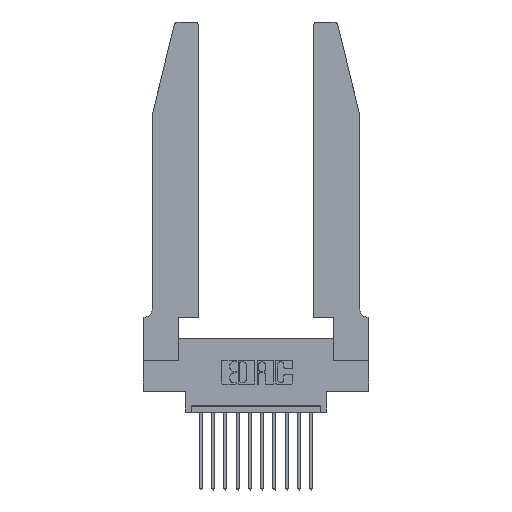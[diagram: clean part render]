
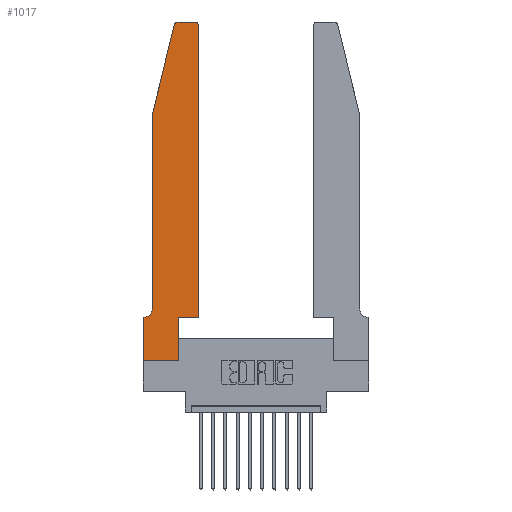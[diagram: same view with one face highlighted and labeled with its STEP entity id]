
A CAD part, top view. The second image highlights one B-rep face of the part: STEP entity #1017.
In plain terms, the highlighted planar face has unit normal (0, 0, 1).
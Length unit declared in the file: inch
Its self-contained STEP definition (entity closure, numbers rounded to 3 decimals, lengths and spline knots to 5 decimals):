
#287 = EDGE_CURVE ( 'NONE', #5123, #6462, #5227, .T. ) ;
#562 = EDGE_CURVE ( 'NONE', #6462, #10882, #5429, .T. ) ;
#591 = LINE ( 'NONE', #732, #14550 ) ;
#655 = LINE ( 'NONE', #1551, #4544 ) ;
#732 = CARTESIAN_POINT ( 'NONE',  ( 0.0755, 2., 0.37 ) ) ;
#905 = ORIENTED_EDGE ( 'NONE', *, *, #12483, .T. ) ;
#939 = ORIENTED_EDGE ( 'NONE', *, *, #8264, .T. ) ;
#1017 = ADVANCED_FACE ( 'NONE', ( #9072 ), #1967, .T. ) ;
#1148 = DIRECTION ( 'NONE',  ( -1., 0., 0. ) ) ;
#1418 = EDGE_CURVE ( 'NONE', #13668, #5212, #11691, .T. ) ;
#1441 = ORIENTED_EDGE ( 'NONE', *, *, #1418, .T. ) ;
#1551 = CARTESIAN_POINT ( 'NONE',  ( 0., 0., 0.37 ) ) ;
#1609 = ORIENTED_EDGE ( 'NONE', *, *, #4348, .T. ) ;
#1967 = PLANE ( 'NONE',  #3558 ) ;
#2048 = CARTESIAN_POINT ( 'NONE',  ( 0.0755, 2., 0.37 ) ) ;
#2219 = EDGE_CURVE ( 'NONE', #9924, #5123, #9487, .T. ) ;
#2852 = DIRECTION ( 'NONE',  ( 0., -1., 0. ) ) ;
#2878 = EDGE_LOOP ( 'NONE', ( #8691, #9067, #11503, #939, #1609, #10460, #5895, #1441, #905, #11869, #11706, #11592 ) ) ;
#2942 = CARTESIAN_POINT ( 'NONE',  ( 0.284, 2.75, 0.37 ) ) ;
#3267 = DIRECTION ( 'NONE',  ( 1., 0., 0. ) ) ;
#3558 = AXIS2_PLACEMENT_3D ( 'NONE', #5874, #7363, #3267 ) ;
#4331 = DIRECTION ( 'NONE',  ( 0., 0., 1. ) ) ;
#4348 = EDGE_CURVE ( 'NONE', #7393, #15270, #9015, .T. ) ;
#4485 = CARTESIAN_POINT ( 'NONE',  ( 0.4505, 0.35, 0.37 ) ) ;
#4508 = DIRECTION ( 'NONE',  ( 1., 0., 0. ) ) ;
#4544 = VECTOR ( 'NONE', #2852, 39.37008 ) ;
#4718 = CARTESIAN_POINT ( 'NONE',  ( 0.0755, 0.35, 0.37 ) ) ;
#4980 = CARTESIAN_POINT ( 'NONE',  ( 0.0055, 0.42, 0.37 ) ) ;
#5123 = VERTEX_POINT ( 'NONE', #12756 ) ;
#5212 = VERTEX_POINT ( 'NONE', #10703 ) ;
#5227 = LINE ( 'NONE', #4485, #16720 ) ;
#5264 = CARTESIAN_POINT ( 'NONE',  ( 0.4205, 2.72, 0.37 ) ) ;
#5366 = CARTESIAN_POINT ( 'NONE',  ( 0., 0.35, 0.37 ) ) ;
#5429 = CIRCLE ( 'NONE', #11139, 0.03 ) ;
#5450 = CARTESIAN_POINT ( 'NONE',  ( 0.2865, 0.35, 0.37 ) ) ;
#5461 = DIRECTION ( 'NONE',  ( 0., 1., 0. ) ) ;
#5874 = CARTESIAN_POINT ( 'NONE',  ( 0., 0.35, 0.37 ) ) ;
#5892 = VERTEX_POINT ( 'NONE', #5366 ) ;
#5895 = ORIENTED_EDGE ( 'NONE', *, *, #12317, .T. ) ;
#6407 = CARTESIAN_POINT ( 'NONE',  ( 0.0055, 0.35, 0.37 ) ) ;
#6462 = VERTEX_POINT ( 'NONE', #16667 ) ;
#6620 = DIRECTION ( 'NONE',  ( -0.239, -0.971, 0. ) ) ;
#6902 = CARTESIAN_POINT ( 'NONE',  ( 0., 0., 0.37 ) ) ;
#7152 = EDGE_CURVE ( 'NONE', #15270, #5892, #15324, .T. ) ;
#7336 = CARTESIAN_POINT ( 'NONE',  ( 0.25487, 2.72718, 0.37 ) ) ;
#7363 = DIRECTION ( 'NONE',  ( 0., 0., 1. ) ) ;
#7393 = VERTEX_POINT ( 'NONE', #14456 ) ;
#7617 = DIRECTION ( 'NONE',  ( 0., 0., -1. ) ) ;
#8003 = DIRECTION ( 'NONE',  ( 1., 0., 0. ) ) ;
#8075 = EDGE_CURVE ( 'NONE', #8812, #16035, #8946, .T. ) ;
#8092 = CARTESIAN_POINT ( 'NONE',  ( 0., 0., 0.37 ) ) ;
#8264 = EDGE_CURVE ( 'NONE', #9399, #7393, #591, .T. ) ;
#8691 = ORIENTED_EDGE ( 'NONE', *, *, #10604, .T. ) ;
#8812 = VERTEX_POINT ( 'NONE', #2942 ) ;
#8946 = CIRCLE ( 'NONE', #13053, 0.03 ) ;
#9015 = CIRCLE ( 'NONE', #10762, 0.07 ) ;
#9067 = ORIENTED_EDGE ( 'NONE', *, *, #8075, .T. ) ;
#9072 = FACE_OUTER_BOUND ( 'NONE', #2878, .T. ) ;
#9260 = CARTESIAN_POINT ( 'NONE',  ( 0.2605, 2.75, 0.37 ) ) ;
#9399 = VERTEX_POINT ( 'NONE', #2048 ) ;
#9463 = DIRECTION ( 'NONE',  ( 1., 0., 0. ) ) ;
#9487 = LINE ( 'NONE', #11033, #12653 ) ;
#9632 = VECTOR ( 'NONE', #5461, 39.37008 ) ;
#9708 = CARTESIAN_POINT ( 'NONE',  ( 0.2865, 0.35, 0.37 ) ) ;
#9923 = VECTOR ( 'NONE', #1148, 39.37008 ) ;
#9924 = VERTEX_POINT ( 'NONE', #5450 ) ;
#10460 = ORIENTED_EDGE ( 'NONE', *, *, #7152, .T. ) ;
#10462 = CARTESIAN_POINT ( 'NONE',  ( 0.0755, 2., 0.37 ) ) ;
#10604 = EDGE_CURVE ( 'NONE', #10882, #8812, #16294, .T. ) ;
#10703 = CARTESIAN_POINT ( 'NONE',  ( 0.2865, 0., 0.37 ) ) ;
#10762 = AXIS2_PLACEMENT_3D ( 'NONE', #4980, #7617, #16587 ) ;
#10882 = VERTEX_POINT ( 'NONE', #13721 ) ;
#11033 = CARTESIAN_POINT ( 'NONE',  ( 0.4505, 0.35, 0.37 ) ) ;
#11060 = LINE ( 'NONE', #10462, #11853 ) ;
#11139 = AXIS2_PLACEMENT_3D ( 'NONE', #5264, #14405, #8003 ) ;
#11503 = ORIENTED_EDGE ( 'NONE', *, *, #16182, .T. ) ;
#11592 = ORIENTED_EDGE ( 'NONE', *, *, #562, .T. ) ;
#11691 = LINE ( 'NONE', #8092, #13109 ) ;
#11706 = ORIENTED_EDGE ( 'NONE', *, *, #287, .T. ) ;
#11853 = VECTOR ( 'NONE', #6620, 39.37008 ) ;
#11869 = ORIENTED_EDGE ( 'NONE', *, *, #2219, .T. ) ;
#12066 = CARTESIAN_POINT ( 'NONE',  ( 0.284, 2.72, 0.37 ) ) ;
#12067 = VECTOR ( 'NONE', #15737, 39.37008 ) ;
#12317 = EDGE_CURVE ( 'NONE', #5892, #13668, #655, .T. ) ;
#12483 = EDGE_CURVE ( 'NONE', #5212, #9924, #15040, .T. ) ;
#12653 = VECTOR ( 'NONE', #4508, 39.37008 ) ;
#12756 = CARTESIAN_POINT ( 'NONE',  ( 0.4505, 0.35, 0.37 ) ) ;
#13053 = AXIS2_PLACEMENT_3D ( 'NONE', #12066, #4331, #14599 ) ;
#13109 = VECTOR ( 'NONE', #9463, 39.37008 ) ;
#13668 = VERTEX_POINT ( 'NONE', #6902 ) ;
#13692 = DIRECTION ( 'NONE',  ( 0., 1., 0. ) ) ;
#13721 = CARTESIAN_POINT ( 'NONE',  ( 0.4205, 2.75, 0.37 ) ) ;
#14405 = DIRECTION ( 'NONE',  ( 0., 0., 1. ) ) ;
#14456 = CARTESIAN_POINT ( 'NONE',  ( 0.0755, 0.42, 0.37 ) ) ;
#14550 = VECTOR ( 'NONE', #15041, 39.37008 ) ;
#14599 = DIRECTION ( 'NONE',  ( 1., 0., 0. ) ) ;
#15040 = LINE ( 'NONE', #9708, #9632 ) ;
#15041 = DIRECTION ( 'NONE',  ( 0., -1., 0. ) ) ;
#15270 = VERTEX_POINT ( 'NONE', #6407 ) ;
#15324 = LINE ( 'NONE', #4718, #9923 ) ;
#15737 = DIRECTION ( 'NONE',  ( -1., 0., 0. ) ) ;
#16035 = VERTEX_POINT ( 'NONE', #7336 ) ;
#16182 = EDGE_CURVE ( 'NONE', #16035, #9399, #11060, .T. ) ;
#16294 = LINE ( 'NONE', #9260, #12067 ) ;
#16587 = DIRECTION ( 'NONE',  ( -1., 0., 0. ) ) ;
#16667 = CARTESIAN_POINT ( 'NONE',  ( 0.4505, 2.72, 0.37 ) ) ;
#16720 = VECTOR ( 'NONE', #13692, 39.37008 ) ;
